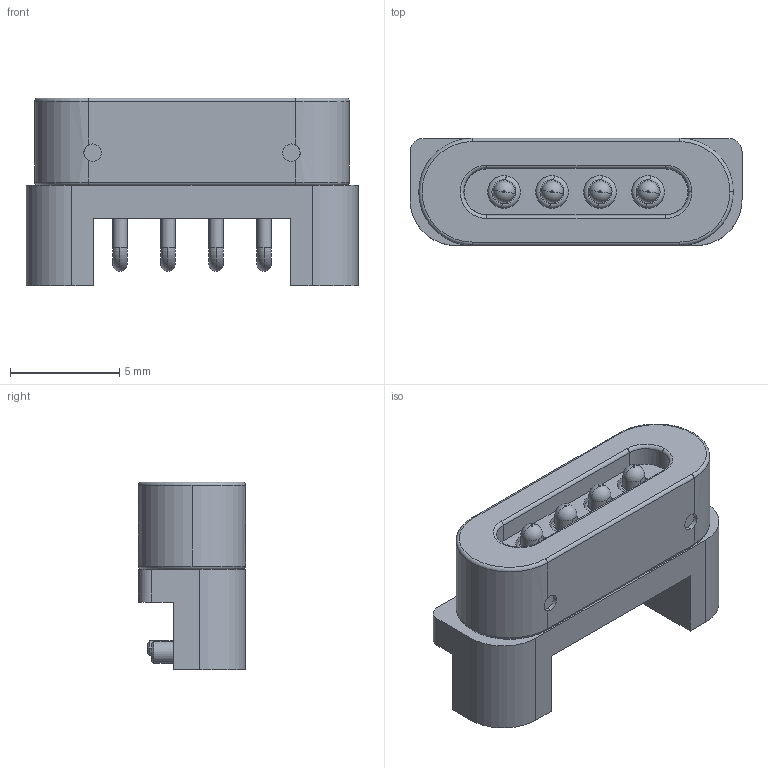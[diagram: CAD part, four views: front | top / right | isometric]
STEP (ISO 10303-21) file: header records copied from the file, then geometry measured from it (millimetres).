
FILE_DESCRIPTION (( 'STEP AP214' ), '1' );
FILE_NAME ('685F0422350125E.STEP', '2023-04-25T18:52:36', ( '' ), ( '' ), 'SwSTEP 2.0', 'SolidWorks 2020', '' );
FILE_SCHEMA (( 'AUTOMOTIVE_DESIGN' ));
Length unit declared in the file: millimetre
Products named in the file (1): 685F0422350125E
Bounding box: 15.2 x 4.9 x 8.6 mm (x, y, z)
Volume: 412.4 mm3; surface area: 658.1 mm2
Topology: 1 solids, 1 shells, 196 faces, 471 edges, 300 vertices
Faces by surface type: cylinder 97, plane 47, torus 28, cone 16, sphere 8
Entity records: 8410 total; most frequent: CARTESIAN_POINT 1411, DIRECTION 1128, ORIENTED_EDGE 942, AXIS2_PLACEMENT_3D 481, EDGE_CURVE 471, VERTEX_POINT 300, CIRCLE 284, EDGE_LOOP 227
